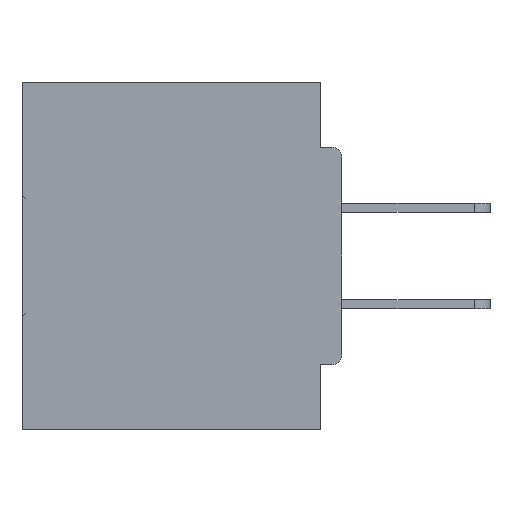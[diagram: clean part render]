
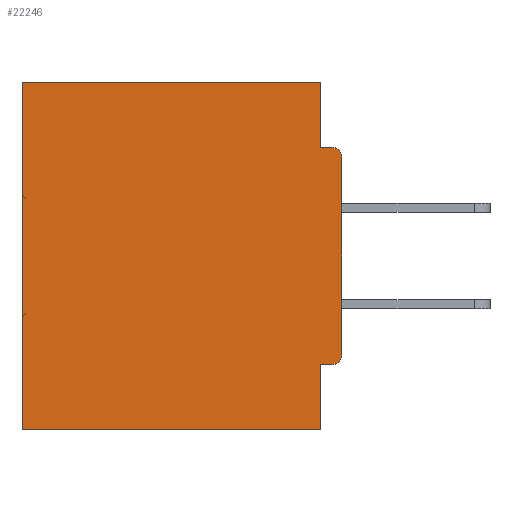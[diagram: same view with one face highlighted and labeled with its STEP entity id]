
A CAD part, left-side view. The second image highlights one B-rep face of the part: STEP entity #22246.
In plain terms, the highlighted planar face has unit normal (-1, 0, 0).
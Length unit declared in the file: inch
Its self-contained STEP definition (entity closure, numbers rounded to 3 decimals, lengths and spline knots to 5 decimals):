
#325 = ORIENTED_EDGE ( 'NONE', *, *, #18445, .F. ) ;
#372 = CARTESIAN_POINT ( 'NONE',  ( 0.298, 0.031, 0. ) ) ;
#549 = CARTESIAN_POINT ( 'NONE',  ( 0.298, 0., -0.3915 ) ) ;
#729 = CARTESIAN_POINT ( 'NONE',  ( 0.298, 0.46, -0.5 ) ) ;
#1143 = CARTESIAN_POINT ( 'NONE',  ( 0.298, 0., 0. ) ) ;
#1285 = VERTEX_POINT ( 'NONE', #729 ) ;
#2529 = VECTOR ( 'NONE', #27379, 39.37008 ) ;
#2545 = CARTESIAN_POINT ( 'NONE',  ( 0.298, 0., -0.5 ) ) ;
#3236 = EDGE_LOOP ( 'NONE', ( #13313, #40432, #7836, #13207, #27433, #325, #15631, #44599, #23426, #37920 ) ) ;
#4045 = DIRECTION ( 'NONE',  ( 1., 0., 0. ) ) ;
#4583 = VERTEX_POINT ( 'NONE', #549 ) ;
#4700 = CARTESIAN_POINT ( 'NONE',  ( 0.298, 0., -0.0935 ) ) ;
#4832 = EDGE_CURVE ( 'NONE', #11339, #4583, #5546, .T. ) ;
#5546 = LINE ( 'NONE', #1143, #12256 ) ;
#7836 = ORIENTED_EDGE ( 'NONE', *, *, #29884, .F. ) ;
#8218 = AXIS2_PLACEMENT_3D ( 'NONE', #25361, #4045, #28897 ) ;
#8349 = CARTESIAN_POINT ( 'NONE',  ( 0.298, 0., -0.4065 ) ) ;
#8489 = VERTEX_POINT ( 'NONE', #20299 ) ;
#9969 = VECTOR ( 'NONE', #18537, 39.37008 ) ;
#10600 = CARTESIAN_POINT ( 'NONE',  ( 0.298, 0., -0.1085 ) ) ;
#11216 = VERTEX_POINT ( 'NONE', #22329 ) ;
#11339 = VERTEX_POINT ( 'NONE', #10600 ) ;
#12204 = DIRECTION ( 'NONE',  ( 0., 0., -1. ) ) ;
#12256 = VECTOR ( 'NONE', #39774, 39.37008 ) ;
#12845 = EDGE_CURVE ( 'NONE', #35601, #8489, #44746, .T. ) ;
#13207 = ORIENTED_EDGE ( 'NONE', *, *, #39209, .T. ) ;
#13313 = ORIENTED_EDGE ( 'NONE', *, *, #15068, .T. ) ;
#14733 = DIRECTION ( 'NONE',  ( -1., 0., 0. ) ) ;
#15028 = CARTESIAN_POINT ( 'NONE',  ( 0.298, 0.015, -0.1085 ) ) ;
#15068 = EDGE_CURVE ( 'NONE', #11339, #31544, #39530, .T. ) ;
#15369 = DIRECTION ( 'NONE',  ( -1., 0., 0. ) ) ;
#15571 = VERTEX_POINT ( 'NONE', #43137 ) ;
#15631 = ORIENTED_EDGE ( 'NONE', *, *, #44683, .F. ) ;
#16505 = DIRECTION ( 'NONE',  ( 0., 0., -1. ) ) ;
#16856 = CIRCLE ( 'NONE', #37515, 0.015 ) ;
#18445 = EDGE_CURVE ( 'NONE', #34758, #1285, #22575, .T. ) ;
#18537 = DIRECTION ( 'NONE',  ( 0., 0., -1. ) ) ;
#20299 = CARTESIAN_POINT ( 'NONE',  ( 0.298, 0.031, -0.4065 ) ) ;
#20775 = DIRECTION ( 'NONE',  ( 0., 1., 0. ) ) ;
#21431 = VERTEX_POINT ( 'NONE', #372 ) ;
#21840 = PLANE ( 'NONE',  #8218 ) ;
#22224 = LINE ( 'NONE', #42746, #9969 ) ;
#22246 = ADVANCED_FACE ( 'NONE', ( #37660 ), #21840, .F. ) ;
#22329 = CARTESIAN_POINT ( 'NONE',  ( 0.298, 0.46, 0. ) ) ;
#22575 = LINE ( 'NONE', #2545, #2529 ) ;
#23426 = ORIENTED_EDGE ( 'NONE', *, *, #37152, .T. ) ;
#24588 = VECTOR ( 'NONE', #12204, 39.37008 ) ;
#25361 = CARTESIAN_POINT ( 'NONE',  ( 0.298, 0., 0. ) ) ;
#25900 = EDGE_CURVE ( 'NONE', #11216, #1285, #44595, .T. ) ;
#25923 = DIRECTION ( 'NONE',  ( 0., 0., -1. ) ) ;
#26075 = CARTESIAN_POINT ( 'NONE',  ( 0.298, 0.015, -0.3915 ) ) ;
#26701 = CARTESIAN_POINT ( 'NONE',  ( 0.298, 0.031, -0.5 ) ) ;
#27015 = VECTOR ( 'NONE', #30384, 39.37008 ) ;
#27379 = DIRECTION ( 'NONE',  ( 0., 1., 0. ) ) ;
#27433 = ORIENTED_EDGE ( 'NONE', *, *, #25900, .T. ) ;
#27468 = CARTESIAN_POINT ( 'NONE',  ( 0.298, 0.015, -0.4065 ) ) ;
#28897 = DIRECTION ( 'NONE',  ( 0., 0., -1. ) ) ;
#29222 = VECTOR ( 'NONE', #16505, 39.37008 ) ;
#29291 = DIRECTION ( 'NONE',  ( 0., 0., -1. ) ) ;
#29386 = CARTESIAN_POINT ( 'NONE',  ( 0.298, 0.46, 0. ) ) ;
#29540 = DIRECTION ( 'NONE',  ( 0., -1., 0. ) ) ;
#29809 = LINE ( 'NONE', #26701, #29222 ) ;
#29884 = EDGE_CURVE ( 'NONE', #21431, #15571, #29809, .T. ) ;
#30384 = DIRECTION ( 'NONE',  ( 0., 1., 0. ) ) ;
#31544 = VERTEX_POINT ( 'NONE', #40955 ) ;
#33971 = LINE ( 'NONE', #4700, #36735 ) ;
#34333 = VECTOR ( 'NONE', #20775, 39.37008 ) ;
#34758 = VERTEX_POINT ( 'NONE', #44358 ) ;
#35601 = VERTEX_POINT ( 'NONE', #27468 ) ;
#36735 = VECTOR ( 'NONE', #29540, 39.37008 ) ;
#37152 = EDGE_CURVE ( 'NONE', #35601, #4583, #16856, .T. ) ;
#37515 = AXIS2_PLACEMENT_3D ( 'NONE', #26075, #15369, #25923 ) ;
#37660 = FACE_OUTER_BOUND ( 'NONE', #3236, .T. ) ;
#37920 = ORIENTED_EDGE ( 'NONE', *, *, #4832, .F. ) ;
#39209 = EDGE_CURVE ( 'NONE', #21431, #11216, #44968, .T. ) ;
#39530 = CIRCLE ( 'NONE', #42217, 0.015 ) ;
#39774 = DIRECTION ( 'NONE',  ( 0., 0., -1. ) ) ;
#40432 = ORIENTED_EDGE ( 'NONE', *, *, #42352, .F. ) ;
#40955 = CARTESIAN_POINT ( 'NONE',  ( 0.298, 0.015, -0.0935 ) ) ;
#41981 = CARTESIAN_POINT ( 'NONE',  ( 0.298, 0., 0. ) ) ;
#42217 = AXIS2_PLACEMENT_3D ( 'NONE', #15028, #14733, #29291 ) ;
#42352 = EDGE_CURVE ( 'NONE', #15571, #31544, #33971, .T. ) ;
#42746 = CARTESIAN_POINT ( 'NONE',  ( 0.298, 0.031, -0.5 ) ) ;
#43137 = CARTESIAN_POINT ( 'NONE',  ( 0.298, 0.031, -0.0935 ) ) ;
#44358 = CARTESIAN_POINT ( 'NONE',  ( 0.298, 0.031, -0.5 ) ) ;
#44595 = LINE ( 'NONE', #29386, #24588 ) ;
#44599 = ORIENTED_EDGE ( 'NONE', *, *, #12845, .F. ) ;
#44683 = EDGE_CURVE ( 'NONE', #8489, #34758, #22224, .T. ) ;
#44746 = LINE ( 'NONE', #8349, #27015 ) ;
#44968 = LINE ( 'NONE', #41981, #34333 ) ;
